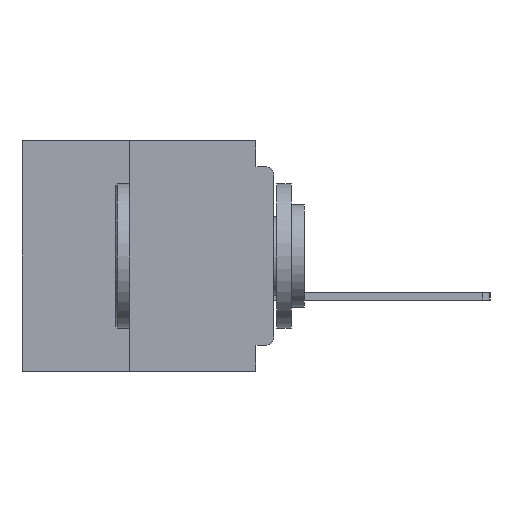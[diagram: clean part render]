
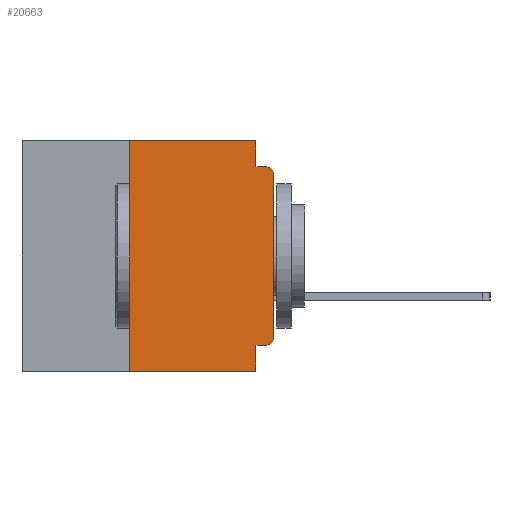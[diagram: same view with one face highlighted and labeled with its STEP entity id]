
A CAD part, left-side view. The second image highlights one B-rep face of the part: STEP entity #20663.
In plain terms, the highlighted planar face has unit normal (-1, 0, 0).
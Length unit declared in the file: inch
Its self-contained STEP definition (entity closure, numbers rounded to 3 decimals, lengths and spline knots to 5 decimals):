
#268 = VERTEX_POINT ( 'NONE', #6238 ) ;
#730 = CARTESIAN_POINT ( 'NONE',  ( 0., 0.015, -0.045 ) ) ;
#897 = ORIENTED_EDGE ( 'NONE', *, *, #18944, .F. ) ;
#1366 = CIRCLE ( 'NONE', #2560, 0.015 ) ;
#1580 = EDGE_CURVE ( 'NONE', #2987, #10118, #11710, .T. ) ;
#2011 = ORIENTED_EDGE ( 'NONE', *, *, #33587, .F. ) ;
#2549 = EDGE_CURVE ( 'NONE', #24638, #11963, #30263, .T. ) ;
#2560 = AXIS2_PLACEMENT_3D ( 'NONE', #3862, #23242, #6664 ) ;
#2746 = PLANE ( 'NONE',  #27767 ) ;
#2987 = VERTEX_POINT ( 'NONE', #20840 ) ;
#3244 = VECTOR ( 'NONE', #29443, 39.37008 ) ;
#3862 = CARTESIAN_POINT ( 'NONE',  ( 0., 0.015, -0.34 ) ) ;
#4262 = DIRECTION ( 'NONE',  ( -1., 0., 0. ) ) ;
#4311 = EDGE_LOOP ( 'NONE', ( #12512, #9093, #16913, #897, #2011, #18625, #35121, #35574, #19928, #4971 ) ) ;
#4971 = ORIENTED_EDGE ( 'NONE', *, *, #6703, .T. ) ;
#5518 = VECTOR ( 'NONE', #25568, 39.37008 ) ;
#6238 = CARTESIAN_POINT ( 'NONE',  ( 0., 0.015, -0.355 ) ) ;
#6664 = DIRECTION ( 'NONE',  ( 0., 0., -1. ) ) ;
#6703 = EDGE_CURVE ( 'NONE', #268, #24638, #1366, .T. ) ;
#8236 = LINE ( 'NONE', #22608, #29456 ) ;
#8343 = DIRECTION ( 'NONE',  ( 0., 0., -1. ) ) ;
#8953 = CARTESIAN_POINT ( 'NONE',  ( 0., 0.031, -0.045 ) ) ;
#9093 = ORIENTED_EDGE ( 'NONE', *, *, #33014, .T. ) ;
#10064 = CARTESIAN_POINT ( 'NONE',  ( 0., 0., -0.355 ) ) ;
#10118 = VERTEX_POINT ( 'NONE', #30094 ) ;
#10394 = VERTEX_POINT ( 'NONE', #730 ) ;
#11710 = LINE ( 'NONE', #16705, #32924 ) ;
#11963 = VERTEX_POINT ( 'NONE', #13236 ) ;
#11977 = FACE_OUTER_BOUND ( 'NONE', #4311, .T. ) ;
#12293 = VECTOR ( 'NONE', #31718, 39.37008 ) ;
#12335 = CARTESIAN_POINT ( 'NONE',  ( 0., 0.031, -0.4 ) ) ;
#12471 = CARTESIAN_POINT ( 'NONE',  ( 0., 0.437, 0. ) ) ;
#12484 = CARTESIAN_POINT ( 'NONE',  ( 0., 0., -0.34 ) ) ;
#12512 = ORIENTED_EDGE ( 'NONE', *, *, #2549, .T. ) ;
#13236 = CARTESIAN_POINT ( 'NONE',  ( 0., 0., -0.06 ) ) ;
#13748 = CARTESIAN_POINT ( 'NONE',  ( 0., 0.031, -0.355 ) ) ;
#14639 = VERTEX_POINT ( 'NONE', #13748 ) ;
#15102 = AXIS2_PLACEMENT_3D ( 'NONE', #20872, #4262, #23660 ) ;
#15306 = LINE ( 'NONE', #12471, #28353 ) ;
#16552 = EDGE_CURVE ( 'NONE', #14639, #29779, #18781, .T. ) ;
#16553 = CARTESIAN_POINT ( 'NONE',  ( 0., 0.437, 0. ) ) ;
#16705 = CARTESIAN_POINT ( 'NONE',  ( 0., 0.25, -0.4 ) ) ;
#16913 = ORIENTED_EDGE ( 'NONE', *, *, #29907, .F. ) ;
#17199 = CARTESIAN_POINT ( 'NONE',  ( 0., 0.437, -0.4 ) ) ;
#17675 = DIRECTION ( 'NONE',  ( 0., 0., 1. ) ) ;
#17783 = VECTOR ( 'NONE', #33381, 39.37008 ) ;
#18625 = ORIENTED_EDGE ( 'NONE', *, *, #1580, .F. ) ;
#18781 = LINE ( 'NONE', #12335, #12293 ) ;
#18944 = EDGE_CURVE ( 'NONE', #25662, #25048, #32521, .T. ) ;
#19928 = ORIENTED_EDGE ( 'NONE', *, *, #26402, .F. ) ;
#20226 = EDGE_CURVE ( 'NONE', #2987, #29779, #28500, .T. ) ;
#20663 = ADVANCED_FACE ( 'NONE', ( #11977 ), #2746, .F. ) ;
#20840 = CARTESIAN_POINT ( 'NONE',  ( 0., 0.25, -0.4 ) ) ;
#20872 = CARTESIAN_POINT ( 'NONE',  ( 0., 0.015, -0.06 ) ) ;
#22608 = CARTESIAN_POINT ( 'NONE',  ( 0., 0., -0.045 ) ) ;
#22723 = DIRECTION ( 'NONE',  ( 0., -1., 0. ) ) ;
#22902 = VECTOR ( 'NONE', #29473, 39.37008 ) ;
#23242 = DIRECTION ( 'NONE',  ( -1., 0., 0. ) ) ;
#23660 = DIRECTION ( 'NONE',  ( 0., 0., -1. ) ) ;
#24638 = VERTEX_POINT ( 'NONE', #12484 ) ;
#24931 = DIRECTION ( 'NONE',  ( 1., 0., 0. ) ) ;
#25048 = VERTEX_POINT ( 'NONE', #8953 ) ;
#25568 = DIRECTION ( 'NONE',  ( 0., -1., 0. ) ) ;
#25662 = VERTEX_POINT ( 'NONE', #28791 ) ;
#26402 = EDGE_CURVE ( 'NONE', #268, #14639, #33576, .T. ) ;
#26626 = CIRCLE ( 'NONE', #15102, 0.015 ) ;
#27767 = AXIS2_PLACEMENT_3D ( 'NONE', #16553, #24931, #8343 ) ;
#27828 = CARTESIAN_POINT ( 'NONE',  ( 0., 0.031, 0. ) ) ;
#28353 = VECTOR ( 'NONE', #34617, 39.37008 ) ;
#28500 = LINE ( 'NONE', #17199, #5518 ) ;
#28791 = CARTESIAN_POINT ( 'NONE',  ( 0., 0.031, 0. ) ) ;
#29443 = DIRECTION ( 'NONE',  ( 0., 1., 0. ) ) ;
#29456 = VECTOR ( 'NONE', #22723, 39.37008 ) ;
#29473 = DIRECTION ( 'NONE',  ( 0., 0., 1. ) ) ;
#29779 = VERTEX_POINT ( 'NONE', #30350 ) ;
#29907 = EDGE_CURVE ( 'NONE', #25048, #10394, #8236, .T. ) ;
#30094 = CARTESIAN_POINT ( 'NONE',  ( 0., 0.25, 0. ) ) ;
#30263 = LINE ( 'NONE', #31188, #22902 ) ;
#30350 = CARTESIAN_POINT ( 'NONE',  ( 0., 0.031, -0.4 ) ) ;
#31188 = CARTESIAN_POINT ( 'NONE',  ( 0., 0., 0. ) ) ;
#31718 = DIRECTION ( 'NONE',  ( 0., 0., -1. ) ) ;
#32521 = LINE ( 'NONE', #27828, #17783 ) ;
#32924 = VECTOR ( 'NONE', #17675, 39.37008 ) ;
#33014 = EDGE_CURVE ( 'NONE', #11963, #10394, #26626, .T. ) ;
#33381 = DIRECTION ( 'NONE',  ( 0., 0., -1. ) ) ;
#33576 = LINE ( 'NONE', #10064, #3244 ) ;
#33587 = EDGE_CURVE ( 'NONE', #10118, #25662, #15306, .T. ) ;
#34617 = DIRECTION ( 'NONE',  ( 0., -1., 0. ) ) ;
#35121 = ORIENTED_EDGE ( 'NONE', *, *, #20226, .T. ) ;
#35574 = ORIENTED_EDGE ( 'NONE', *, *, #16552, .F. ) ;
